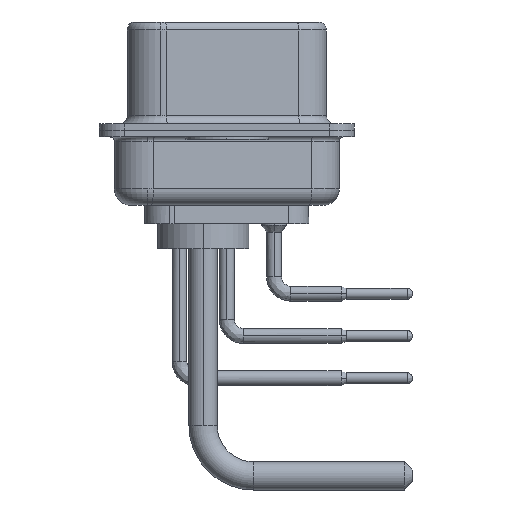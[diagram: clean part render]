
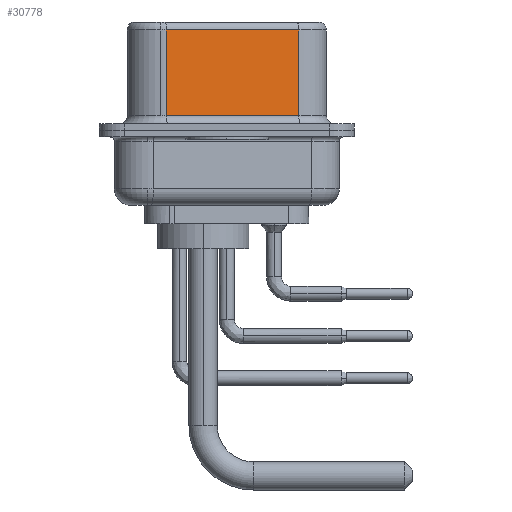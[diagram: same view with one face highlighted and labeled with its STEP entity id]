
A CAD part, left-side view. The second image highlights one B-rep face of the part: STEP entity #30778.
In plain terms, the highlighted planar face has unit normal (-0.985, -0.174, 0).
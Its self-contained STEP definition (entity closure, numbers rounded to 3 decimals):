
#1167 = VERTEX_POINT ( 'NONE', #9724 ) ;
#1242 = PLANE ( 'NONE',  #29332 ) ;
#1557 = DIRECTION ( 'NONE',  ( 0.985, 0.174, 0. ) ) ;
#1955 = CARTESIAN_POINT ( 'NONE',  ( 3.73, 3.628, 6.52 ) ) ;
#5934 = VERTEX_POINT ( 'NONE', #15491 ) ;
#6483 = CARTESIAN_POINT ( 'NONE',  ( 5.132, -4.322, 6.52 ) ) ;
#7155 = LINE ( 'NONE', #19787, #13232 ) ;
#7354 = LINE ( 'NONE', #11617, #18826 ) ;
#7557 = EDGE_CURVE ( 'NONE', #19167, #1167, #7155, .T. ) ;
#9724 = CARTESIAN_POINT ( 'NONE',  ( 5.132, -4.322, 0.9 ) ) ;
#9861 = LINE ( 'NONE', #27421, #21712 ) ;
#10103 = EDGE_CURVE ( 'NONE', #26590, #19167, #21967, .T. ) ;
#11617 = CARTESIAN_POINT ( 'NONE',  ( 5.132, -4.322, 6.52 ) ) ;
#13165 = EDGE_LOOP ( 'NONE', ( #30511, #18747, #25423, #31467 ) ) ;
#13232 = VECTOR ( 'NONE', #29780, 1000. ) ;
#14842 = CARTESIAN_POINT ( 'NONE',  ( 3.73, 3.628, 0.9 ) ) ;
#14849 = EDGE_CURVE ( 'NONE', #5934, #1167, #7354, .T. ) ;
#15491 = CARTESIAN_POINT ( 'NONE',  ( 5.132, -4.322, 6.02 ) ) ;
#17437 = DIRECTION ( 'NONE',  ( -0.174, 0.985, 0. ) ) ;
#18747 = ORIENTED_EDGE ( 'NONE', *, *, #25584, .T. ) ;
#18826 = VECTOR ( 'NONE', #24261, 1000. ) ;
#19167 = VERTEX_POINT ( 'NONE', #14842 ) ;
#19787 = CARTESIAN_POINT ( 'NONE',  ( 5.132, -4.322, 0.9 ) ) ;
#21712 = VECTOR ( 'NONE', #17437, 1000. ) ;
#21967 = LINE ( 'NONE', #1955, #29599 ) ;
#22428 = CARTESIAN_POINT ( 'NONE',  ( 3.73, 3.628, 6.02 ) ) ;
#24261 = DIRECTION ( 'NONE',  ( 0., 0., -1. ) ) ;
#25423 = ORIENTED_EDGE ( 'NONE', *, *, #10103, .T. ) ;
#25584 = EDGE_CURVE ( 'NONE', #5934, #26590, #9861, .T. ) ;
#26590 = VERTEX_POINT ( 'NONE', #22428 ) ;
#27421 = CARTESIAN_POINT ( 'NONE',  ( 5.132, -4.322, 6.02 ) ) ;
#29332 = AXIS2_PLACEMENT_3D ( 'NONE', #6483, #1557, #31566 ) ;
#29599 = VECTOR ( 'NONE', #29992, 1000. ) ;
#29780 = DIRECTION ( 'NONE',  ( 0.174, -0.985, 0. ) ) ;
#29992 = DIRECTION ( 'NONE',  ( 0., 0., -1. ) ) ;
#30482 = FACE_OUTER_BOUND ( 'NONE', #13165, .T. ) ;
#30511 = ORIENTED_EDGE ( 'NONE', *, *, #14849, .F. ) ;
#30778 = ADVANCED_FACE ( 'NONE', ( #30482 ), #1242, .F. ) ;
#31467 = ORIENTED_EDGE ( 'NONE', *, *, #7557, .T. ) ;
#31566 = DIRECTION ( 'NONE',  ( -0.174, 0.985, 0. ) ) ;
